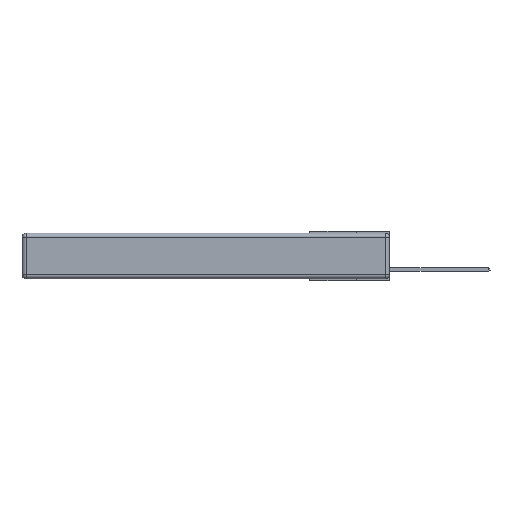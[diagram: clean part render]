
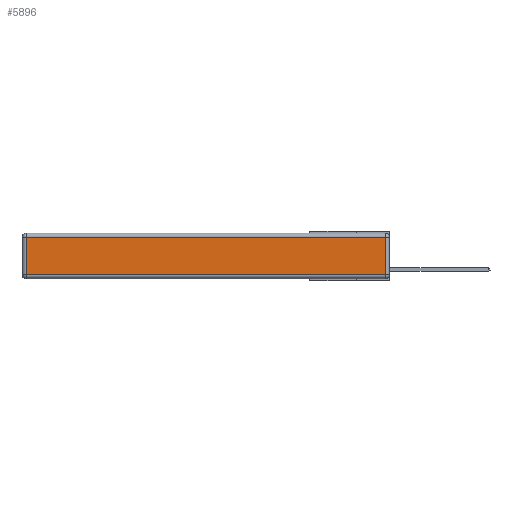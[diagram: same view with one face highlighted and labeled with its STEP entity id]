
A CAD part, left-side view. The second image highlights one B-rep face of the part: STEP entity #5896.
In plain terms, the highlighted planar face has unit normal (-1, 0, 0).
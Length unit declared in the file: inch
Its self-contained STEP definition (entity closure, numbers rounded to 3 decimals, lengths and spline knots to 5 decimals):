
#658 = FACE_OUTER_BOUND ( 'NONE', #9568, .T. ) ;
#791 = DIRECTION ( 'NONE',  ( 0., 0., -1. ) ) ;
#803 = CARTESIAN_POINT ( 'NONE',  ( 0., 2.72, -0.03 ) ) ;
#1843 = DIRECTION ( 'NONE',  ( 0., 1., 0. ) ) ;
#2054 = CARTESIAN_POINT ( 'NONE',  ( 0., 0.03, -0.03 ) ) ;
#2087 = CARTESIAN_POINT ( 'NONE',  ( 0., 0.03, -0.343 ) ) ;
#2105 = CARTESIAN_POINT ( 'NONE',  ( 0., 0., -0.313 ) ) ;
#2133 = LINE ( 'NONE', #12820, #2483 ) ;
#2483 = VECTOR ( 'NONE', #791, 39.37008 ) ;
#2846 = CARTESIAN_POINT ( 'NONE',  ( 0., 2.75, -0.03 ) ) ;
#2907 = LINE ( 'NONE', #2087, #10693 ) ;
#2915 = AXIS2_PLACEMENT_3D ( 'NONE', #11771, #7385, #10581 ) ;
#2950 = EDGE_CURVE ( 'NONE', #8379, #5230, #2133, .T. ) ;
#4489 = DIRECTION ( 'NONE',  ( 0., -1., 0. ) ) ;
#5230 = VERTEX_POINT ( 'NONE', #11211 ) ;
#5252 = VERTEX_POINT ( 'NONE', #2054 ) ;
#5881 = LINE ( 'NONE', #2105, #6735 ) ;
#5896 = ADVANCED_FACE ( 'NONE', ( #658 ), #12764, .T. ) ;
#6116 = VECTOR ( 'NONE', #1843, 39.37008 ) ;
#6717 = CARTESIAN_POINT ( 'NONE',  ( 0., 0.03, -0.313 ) ) ;
#6735 = VECTOR ( 'NONE', #4489, 39.37008 ) ;
#6880 = VERTEX_POINT ( 'NONE', #6717 ) ;
#7385 = DIRECTION ( 'NONE',  ( -1., 0., 0. ) ) ;
#7535 = DIRECTION ( 'NONE',  ( 0., 0., 1. ) ) ;
#8279 = EDGE_CURVE ( 'NONE', #5230, #6880, #5881, .T. ) ;
#8379 = VERTEX_POINT ( 'NONE', #803 ) ;
#9010 = ORIENTED_EDGE ( 'NONE', *, *, #12305, .T. ) ;
#9242 = ORIENTED_EDGE ( 'NONE', *, *, #2950, .T. ) ;
#9398 = LINE ( 'NONE', #2846, #6116 ) ;
#9568 = EDGE_LOOP ( 'NONE', ( #12333, #14378, #9010, #9242 ) ) ;
#9611 = EDGE_CURVE ( 'NONE', #6880, #5252, #2907, .T. ) ;
#10581 = DIRECTION ( 'NONE',  ( 0., 0., 1. ) ) ;
#10693 = VECTOR ( 'NONE', #7535, 39.37008 ) ;
#11211 = CARTESIAN_POINT ( 'NONE',  ( 0., 2.72, -0.313 ) ) ;
#11771 = CARTESIAN_POINT ( 'NONE',  ( 0., 0., -0.343 ) ) ;
#12305 = EDGE_CURVE ( 'NONE', #5252, #8379, #9398, .T. ) ;
#12333 = ORIENTED_EDGE ( 'NONE', *, *, #8279, .T. ) ;
#12764 = PLANE ( 'NONE',  #2915 ) ;
#12820 = CARTESIAN_POINT ( 'NONE',  ( 0., 2.72, -0.343 ) ) ;
#14378 = ORIENTED_EDGE ( 'NONE', *, *, #9611, .T. ) ;
